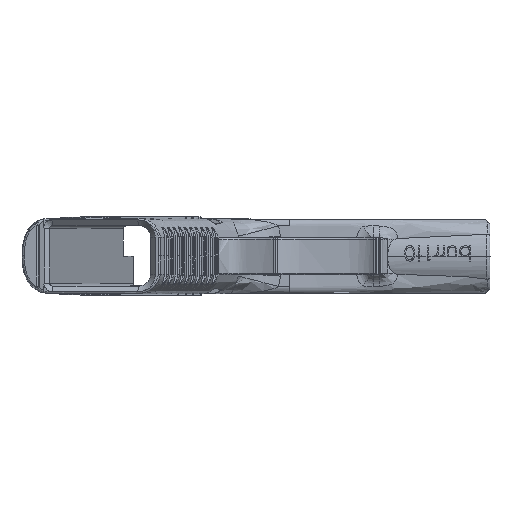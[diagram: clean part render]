
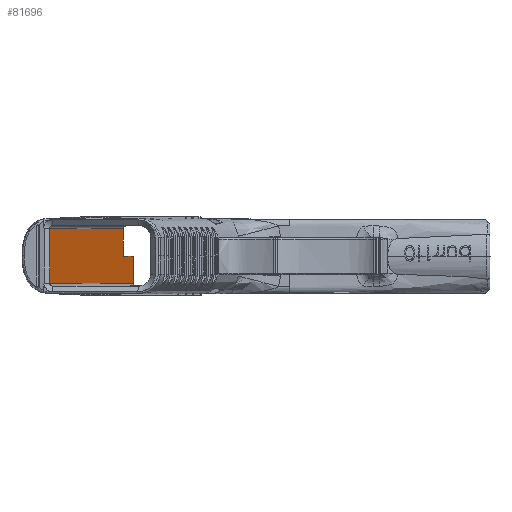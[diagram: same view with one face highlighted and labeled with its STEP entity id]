
A CAD part, top view. The second image highlights one B-rep face of the part: STEP entity #81696.
In plain terms, the highlighted planar face has unit normal (0.951, 0, 0.309).
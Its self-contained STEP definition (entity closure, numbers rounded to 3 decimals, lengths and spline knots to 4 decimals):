
#5772 = ORIENTED_EDGE ( 'NONE', *, *, #25768, .F. ) ;
#25768 = EDGE_CURVE ( 'NONE', #269429, #296270, #363972, .T. ) ;
#28819 = LINE ( 'NONE', #104126, #219681 ) ;
#38864 = EDGE_CURVE ( 'NONE', #218910, #363017, #214766, .T. ) ;
#55454 = LINE ( 'NONE', #189001, #65008 ) ;
#65008 = VECTOR ( 'NONE', #95750, 39.3701 ) ;
#74965 = EDGE_CURVE ( 'NONE', #254213, #134404, #322366, .T. ) ;
#81696 = ADVANCED_FACE ( 'NONE', ( #235589 ), #321463, .F. ) ;
#82968 = EDGE_CURVE ( 'NONE', #296270, #254213, #116344, .T. ) ;
#95750 = DIRECTION ( 'NONE',  ( -0.309, 0., 0.951 ) ) ;
#104126 = CARTESIAN_POINT ( 'NONE',  ( 2.0746, 0.0001, -3.8765 ) ) ;
#115998 = CARTESIAN_POINT ( 'NONE',  ( 1.9466, 0.0001, -3.4826 ) ) ;
#116344 = LINE ( 'NONE', #299916, #154549 ) ;
#134404 = VERTEX_POINT ( 'NONE', #115998 ) ;
#154549 = VECTOR ( 'NONE', #154816, 39.3701 ) ;
#154816 = DIRECTION ( 'NONE',  ( 0.309, 0., -0.951 ) ) ;
#160793 = DIRECTION ( 'NONE',  ( 0., 1., 0. ) ) ;
#167305 = VECTOR ( 'NONE', #231862, 39.3701 ) ;
#186357 = CARTESIAN_POINT ( 'NONE',  ( 0.9499, 0.37, -0.4151 ) ) ;
#189001 = CARTESIAN_POINT ( 'NONE',  ( 2.0746, -0.37, -3.8765 ) ) ;
#203108 = VECTOR ( 'NONE', #306695, 39.3701 ) ;
#214766 = LINE ( 'NONE', #287868, #167305 ) ;
#217657 = CARTESIAN_POINT ( 'NONE',  ( 0.9499, -0.37, -0.4151 ) ) ;
#218910 = VERTEX_POINT ( 'NONE', #336853 ) ;
#219681 = VECTOR ( 'NONE', #319902, 39.3701 ) ;
#231862 = DIRECTION ( 'NONE',  ( 0., -1., 0. ) ) ;
#235589 = FACE_OUTER_BOUND ( 'NONE', #275216, .T. ) ;
#254213 = VERTEX_POINT ( 'NONE', #314209 ) ;
#266875 = CARTESIAN_POINT ( 'NONE',  ( 1.9466, 0., -3.4826 ) ) ;
#269429 = VERTEX_POINT ( 'NONE', #217657 ) ;
#275216 = EDGE_LOOP ( 'NONE', ( #325208, #314165, #5772, #314753, #318403, #354358 ) ) ;
#282761 = VECTOR ( 'NONE', #160793, 39.3701 ) ;
#287240 = CARTESIAN_POINT ( 'NONE',  ( 0.9499, 0., -0.4151 ) ) ;
#287868 = CARTESIAN_POINT ( 'NONE',  ( 2.0809, 0., -3.896 ) ) ;
#296270 = VERTEX_POINT ( 'NONE', #186357 ) ;
#296512 = EDGE_CURVE ( 'NONE', #363017, #269429, #55454, .T. ) ;
#299916 = CARTESIAN_POINT ( 'NONE',  ( 2.0746, 0.37, -3.8765 ) ) ;
#306695 = DIRECTION ( 'NONE',  ( 0., -1., 0. ) ) ;
#307408 = CARTESIAN_POINT ( 'NONE',  ( 2.0809, -0.37, -3.896 ) ) ;
#314165 = ORIENTED_EDGE ( 'NONE', *, *, #82968, .F. ) ;
#314209 = CARTESIAN_POINT ( 'NONE',  ( 1.9466, 0.37, -3.4826 ) ) ;
#314753 = ORIENTED_EDGE ( 'NONE', *, *, #296512, .F. ) ;
#318403 = ORIENTED_EDGE ( 'NONE', *, *, #38864, .F. ) ;
#319902 = DIRECTION ( 'NONE',  ( 0.309, 0., -0.951 ) ) ;
#321463 = PLANE ( 'NONE',  #375073 ) ;
#322366 = LINE ( 'NONE', #266875, #203108 ) ;
#325208 = ORIENTED_EDGE ( 'NONE', *, *, #74965, .F. ) ;
#336853 = CARTESIAN_POINT ( 'NONE',  ( 2.0809, 0.0001, -3.896 ) ) ;
#352171 = DIRECTION ( 'NONE',  ( -0.951, 0., -0.309 ) ) ;
#354358 = ORIENTED_EDGE ( 'NONE', *, *, #373745, .F. ) ;
#363017 = VERTEX_POINT ( 'NONE', #307408 ) ;
#363972 = LINE ( 'NONE', #287240, #282761 ) ;
#373745 = EDGE_CURVE ( 'NONE', #134404, #218910, #28819, .T. ) ;
#375073 = AXIS2_PLACEMENT_3D ( 'NONE', #381539, #352171, #378922 ) ;
#378922 = DIRECTION ( 'NONE',  ( -0.309, 0., 0.951 ) ) ;
#381539 = CARTESIAN_POINT ( 'NONE',  ( 2.0746, 0., -3.8765 ) ) ;
